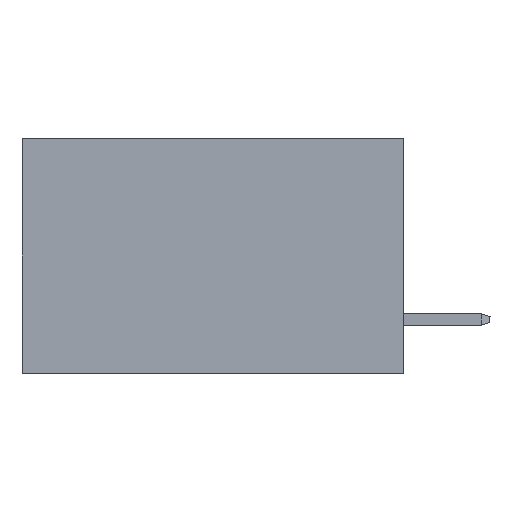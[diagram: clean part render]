
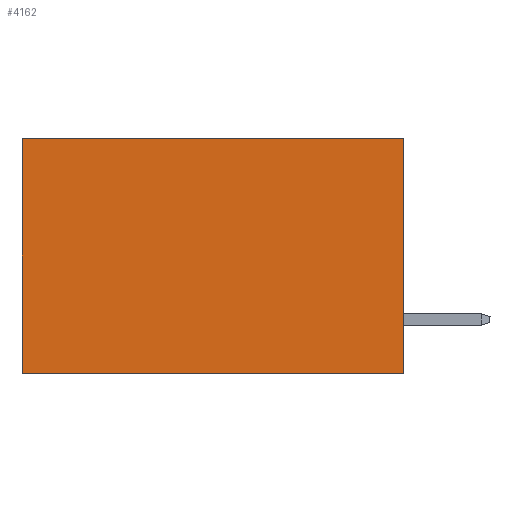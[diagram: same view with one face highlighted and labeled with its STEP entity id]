
A CAD part, left-side view. The second image highlights one B-rep face of the part: STEP entity #4162.
In plain terms, the highlighted planar face has unit normal (-1, 0, 0).
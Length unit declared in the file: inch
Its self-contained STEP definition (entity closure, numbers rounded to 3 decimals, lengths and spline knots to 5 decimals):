
#614 = VECTOR ( 'NONE', #4712, 39.37008 ) ;
#780 = DIRECTION ( 'NONE',  ( 0., 0., -1. ) ) ;
#1914 = CARTESIAN_POINT ( 'NONE',  ( 0.2875, 0., -0.37 ) ) ;
#2079 = VERTEX_POINT ( 'NONE', #13533 ) ;
#2865 = ORIENTED_EDGE ( 'NONE', *, *, #14711, .F. ) ;
#3936 = VECTOR ( 'NONE', #780, 39.37008 ) ;
#4162 = ADVANCED_FACE ( 'NONE', ( #15664 ), #14052, .F. ) ;
#4712 = DIRECTION ( 'NONE',  ( 0., 1., 0. ) ) ;
#5339 = VERTEX_POINT ( 'NONE', #10885 ) ;
#6198 = LINE ( 'NONE', #7832, #614 ) ;
#6622 = ORIENTED_EDGE ( 'NONE', *, *, #11851, .T. ) ;
#6739 = LINE ( 'NONE', #1914, #11039 ) ;
#6811 = DIRECTION ( 'NONE',  ( 1., 0., 0. ) ) ;
#7162 = DIRECTION ( 'NONE',  ( 0., 0., -1. ) ) ;
#7513 = ORIENTED_EDGE ( 'NONE', *, *, #11409, .T. ) ;
#7832 = CARTESIAN_POINT ( 'NONE',  ( 0.2875, 0., 0. ) ) ;
#8245 = LINE ( 'NONE', #11456, #3936 ) ;
#8593 = AXIS2_PLACEMENT_3D ( 'NONE', #15544, #6811, #7162 ) ;
#8919 = DIRECTION ( 'NONE',  ( 0., 1., 0. ) ) ;
#8984 = CARTESIAN_POINT ( 'NONE',  ( 0.2875, 0., 0. ) ) ;
#10885 = CARTESIAN_POINT ( 'NONE',  ( 0.2875, 0., -0.37 ) ) ;
#11039 = VECTOR ( 'NONE', #8919, 39.37008 ) ;
#11221 = LINE ( 'NONE', #14565, #22418 ) ;
#11409 = EDGE_CURVE ( 'NONE', #16550, #20166, #6198, .T. ) ;
#11456 = CARTESIAN_POINT ( 'NONE',  ( 0.2875, 0.6, 0. ) ) ;
#11851 = EDGE_CURVE ( 'NONE', #20166, #2079, #8245, .T. ) ;
#12499 = EDGE_LOOP ( 'NONE', ( #6622, #15657, #2865, #7513 ) ) ;
#13533 = CARTESIAN_POINT ( 'NONE',  ( 0.2875, 0.6, -0.37 ) ) ;
#14052 = PLANE ( 'NONE',  #8593 ) ;
#14565 = CARTESIAN_POINT ( 'NONE',  ( 0.2875, 0., 0. ) ) ;
#14641 = EDGE_CURVE ( 'NONE', #5339, #2079, #6739, .T. ) ;
#14711 = EDGE_CURVE ( 'NONE', #16550, #5339, #11221, .T. ) ;
#15544 = CARTESIAN_POINT ( 'NONE',  ( 0.2875, 0., 0. ) ) ;
#15657 = ORIENTED_EDGE ( 'NONE', *, *, #14641, .F. ) ;
#15664 = FACE_OUTER_BOUND ( 'NONE', #12499, .T. ) ;
#16550 = VERTEX_POINT ( 'NONE', #8984 ) ;
#17288 = CARTESIAN_POINT ( 'NONE',  ( 0.2875, 0.6, 0. ) ) ;
#18132 = DIRECTION ( 'NONE',  ( 0., 0., -1. ) ) ;
#20166 = VERTEX_POINT ( 'NONE', #17288 ) ;
#22418 = VECTOR ( 'NONE', #18132, 39.37008 ) ;
